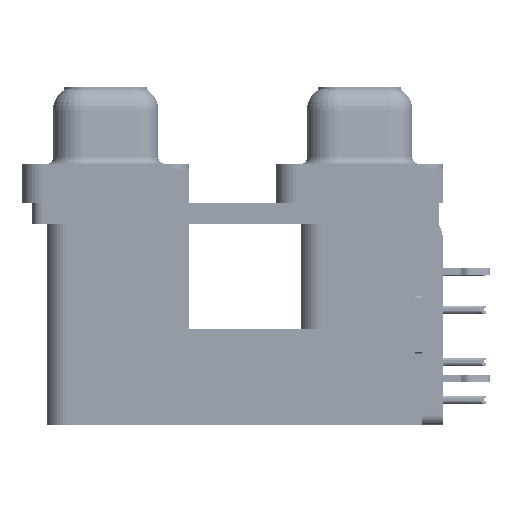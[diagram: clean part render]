
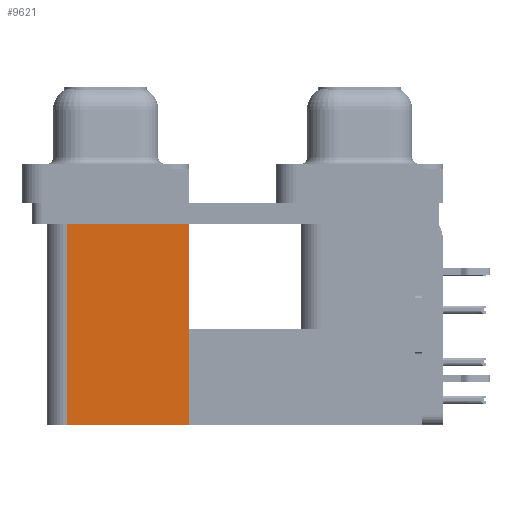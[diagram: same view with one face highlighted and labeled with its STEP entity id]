
A CAD part, left-side view. The second image highlights one B-rep face of the part: STEP entity #9621.
In plain terms, the highlighted planar face has unit normal (-1, 0, 0).
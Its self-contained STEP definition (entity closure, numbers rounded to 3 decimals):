
#191 = LINE ( 'NONE', #44270, #56640 ) ;
#455 = DIRECTION ( 'NONE',  ( 0., 0., 1. ) ) ;
#2003 = PLANE ( 'NONE',  #33939 ) ;
#2327 = CARTESIAN_POINT ( 'NONE',  ( 3.7, 21.975, -19.2 ) ) ;
#3106 = CARTESIAN_POINT ( 'NONE',  ( 3.7, 12.775, -19.2 ) ) ;
#3890 = CARTESIAN_POINT ( 'NONE',  ( 3.7, 12.775, -2.5 ) ) ;
#5190 = EDGE_CURVE ( 'NONE', #9399, #49716, #17056, .T. ) ;
#5679 = VERTEX_POINT ( 'NONE', #31676 ) ;
#6488 = CARTESIAN_POINT ( 'NONE',  ( 3.7, 21.975, -19.2 ) ) ;
#7022 = ORIENTED_EDGE ( 'NONE', *, *, #29791, .F. ) ;
#9399 = VERTEX_POINT ( 'NONE', #6488 ) ;
#9621 = ADVANCED_FACE ( 'NONE', ( #17375 ), #2003, .F. ) ;
#10655 = LINE ( 'NONE', #29871, #36661 ) ;
#11998 = ORIENTED_EDGE ( 'NONE', *, *, #22269, .T. ) ;
#12551 = EDGE_LOOP ( 'NONE', ( #11998, #29048, #7022, #44228 ) ) ;
#17056 = LINE ( 'NONE', #2327, #23112 ) ;
#17375 = FACE_OUTER_BOUND ( 'NONE', #12551, .T. ) ;
#22269 = EDGE_CURVE ( 'NONE', #5679, #49716, #62019, .T. ) ;
#23112 = VECTOR ( 'NONE', #26960, 1000. ) ;
#24523 = VERTEX_POINT ( 'NONE', #3106 ) ;
#26960 = DIRECTION ( 'NONE',  ( 0., 0., 1. ) ) ;
#28816 = VECTOR ( 'NONE', #42874, 1000. ) ;
#29048 = ORIENTED_EDGE ( 'NONE', *, *, #5190, .F. ) ;
#29791 = EDGE_CURVE ( 'NONE', #24523, #9399, #191, .T. ) ;
#29871 = CARTESIAN_POINT ( 'NONE',  ( 3.7, 12.775, -19.2 ) ) ;
#31676 = CARTESIAN_POINT ( 'NONE',  ( 3.7, 12.775, -2.5 ) ) ;
#33939 = AXIS2_PLACEMENT_3D ( 'NONE', #52153, #37147, #56608 ) ;
#36661 = VECTOR ( 'NONE', #455, 1000. ) ;
#37147 = DIRECTION ( 'NONE',  ( 1., 0., 0. ) ) ;
#42121 = CARTESIAN_POINT ( 'NONE',  ( 3.7, 21.975, -2.5 ) ) ;
#42874 = DIRECTION ( 'NONE',  ( 0., 1., 0. ) ) ;
#44228 = ORIENTED_EDGE ( 'NONE', *, *, #56829, .T. ) ;
#44270 = CARTESIAN_POINT ( 'NONE',  ( 3.7, 12.775, -19.2 ) ) ;
#49716 = VERTEX_POINT ( 'NONE', #42121 ) ;
#52153 = CARTESIAN_POINT ( 'NONE',  ( 3.7, 12.775, -19.2 ) ) ;
#56608 = DIRECTION ( 'NONE',  ( 0., 1., 0. ) ) ;
#56640 = VECTOR ( 'NONE', #59856, 1000. ) ;
#56829 = EDGE_CURVE ( 'NONE', #24523, #5679, #10655, .T. ) ;
#59856 = DIRECTION ( 'NONE',  ( 0., 1., 0. ) ) ;
#62019 = LINE ( 'NONE', #3890, #28816 ) ;
